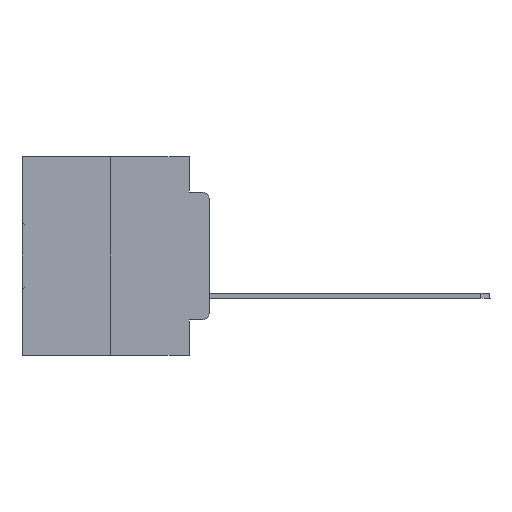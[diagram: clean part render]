
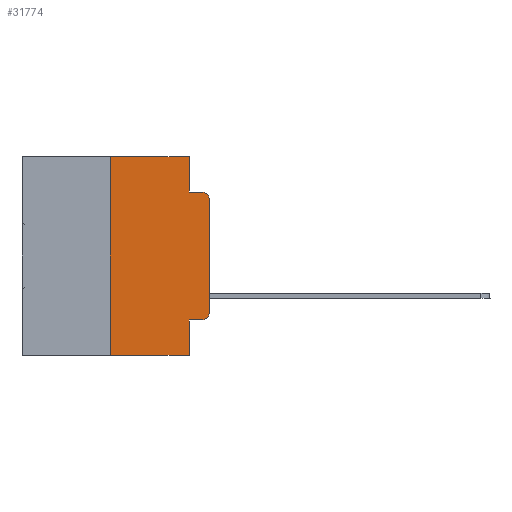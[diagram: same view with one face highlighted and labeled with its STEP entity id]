
A CAD part, left-side view. The second image highlights one B-rep face of the part: STEP entity #31774.
In plain terms, the highlighted planar face has unit normal (-1, 0, 0).
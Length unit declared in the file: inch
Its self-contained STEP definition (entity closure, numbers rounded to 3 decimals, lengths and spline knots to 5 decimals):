
#291 = CARTESIAN_POINT ( 'NONE',  ( 0., 0., -0.3915 ) ) ;
#1511 = EDGE_CURVE ( 'NONE', #17977, #1624, #19729, .T. ) ;
#1624 = VERTEX_POINT ( 'NONE', #20412 ) ;
#1772 = EDGE_LOOP ( 'NONE', ( #11025, #20666, #19394, #4101, #31444, #15307, #18161, #24381, #7701, #19922 ) ) ;
#2603 = CIRCLE ( 'NONE', #23754, 0.02 ) ;
#2684 = DIRECTION ( 'NONE',  ( 0., 0., -1. ) ) ;
#2733 = LINE ( 'NONE', #8627, #13913 ) ;
#2771 = VERTEX_POINT ( 'NONE', #5417 ) ;
#2804 = EDGE_CURVE ( 'NONE', #32951, #7761, #2733, .T. ) ;
#2939 = CARTESIAN_POINT ( 'NONE',  ( 0., 0.051, -0.4115 ) ) ;
#3077 = LINE ( 'NONE', #18173, #30361 ) ;
#3597 = DIRECTION ( 'NONE',  ( 0., -1., 0. ) ) ;
#3791 = CARTESIAN_POINT ( 'NONE',  ( 0., 0.25, 0. ) ) ;
#3848 = CARTESIAN_POINT ( 'NONE',  ( 0., 0.051, -0.5 ) ) ;
#4101 = ORIENTED_EDGE ( 'NONE', *, *, #33173, .F. ) ;
#4115 = CARTESIAN_POINT ( 'NONE',  ( 0., 0.02, -0.1085 ) ) ;
#4470 = FACE_OUTER_BOUND ( 'NONE', #1772, .T. ) ;
#4649 = EDGE_CURVE ( 'NONE', #1624, #17998, #2603, .T. ) ;
#5417 = CARTESIAN_POINT ( 'NONE',  ( 0., 0., -0.1085 ) ) ;
#6479 = LINE ( 'NONE', #16119, #21344 ) ;
#6484 = CARTESIAN_POINT ( 'NONE',  ( 0., 0.25, -0.5 ) ) ;
#6790 = CARTESIAN_POINT ( 'NONE',  ( 0., 0.051, 0. ) ) ;
#7687 = EDGE_CURVE ( 'NONE', #17998, #2771, #6479, .T. ) ;
#7701 = ORIENTED_EDGE ( 'NONE', *, *, #1511, .T. ) ;
#7761 = VERTEX_POINT ( 'NONE', #11433 ) ;
#8071 = VECTOR ( 'NONE', #3597, 39.37008 ) ;
#8291 = VERTEX_POINT ( 'NONE', #18650 ) ;
#8627 = CARTESIAN_POINT ( 'NONE',  ( 0., 0.051, -0.0885 ) ) ;
#9637 = LINE ( 'NONE', #3791, #29026 ) ;
#9749 = DIRECTION ( 'NONE',  ( 1., 0., 0. ) ) ;
#10572 = VECTOR ( 'NONE', #25533, 39.37008 ) ;
#10906 = CARTESIAN_POINT ( 'NONE',  ( 0., 0.02, -0.3915 ) ) ;
#11025 = ORIENTED_EDGE ( 'NONE', *, *, #7687, .T. ) ;
#11335 = AXIS2_PLACEMENT_3D ( 'NONE', #4115, #22582, #27676 ) ;
#11377 = CARTESIAN_POINT ( 'NONE',  ( 0., 0.473, 0. ) ) ;
#11433 = CARTESIAN_POINT ( 'NONE',  ( 0., 0.02, -0.0885 ) ) ;
#12043 = CARTESIAN_POINT ( 'NONE',  ( 0., 0.051, -0.4115 ) ) ;
#12288 = EDGE_CURVE ( 'NONE', #25626, #14626, #3077, .T. ) ;
#12292 = VECTOR ( 'NONE', #2684, 39.37008 ) ;
#13536 = DIRECTION ( 'NONE',  ( 0., 0., -1. ) ) ;
#13904 = EDGE_CURVE ( 'NONE', #25626, #8291, #9637, .T. ) ;
#13913 = VECTOR ( 'NONE', #25048, 39.37008 ) ;
#14626 = VERTEX_POINT ( 'NONE', #3848 ) ;
#15028 = CARTESIAN_POINT ( 'NONE',  ( 0., 0.473, 0. ) ) ;
#15307 = ORIENTED_EDGE ( 'NONE', *, *, #13904, .F. ) ;
#16119 = CARTESIAN_POINT ( 'NONE',  ( 0., 0., 0. ) ) ;
#17690 = DIRECTION ( 'NONE',  ( 0., 0., -1. ) ) ;
#17977 = VERTEX_POINT ( 'NONE', #2939 ) ;
#17998 = VERTEX_POINT ( 'NONE', #291 ) ;
#18161 = ORIENTED_EDGE ( 'NONE', *, *, #12288, .T. ) ;
#18173 = CARTESIAN_POINT ( 'NONE',  ( 0., 0.473, -0.5 ) ) ;
#18650 = CARTESIAN_POINT ( 'NONE',  ( 0., 0.25, 0. ) ) ;
#19394 = ORIENTED_EDGE ( 'NONE', *, *, #2804, .F. ) ;
#19729 = LINE ( 'NONE', #12043, #20132 ) ;
#19922 = ORIENTED_EDGE ( 'NONE', *, *, #4649, .T. ) ;
#20132 = VECTOR ( 'NONE', #24913, 39.37008 ) ;
#20412 = CARTESIAN_POINT ( 'NONE',  ( 0., 0.02, -0.4115 ) ) ;
#20666 = ORIENTED_EDGE ( 'NONE', *, *, #25065, .T. ) ;
#21001 = CIRCLE ( 'NONE', #11335, 0.02 ) ;
#21130 = AXIS2_PLACEMENT_3D ( 'NONE', #15028, #9749, #17690 ) ;
#21344 = VECTOR ( 'NONE', #28986, 39.37008 ) ;
#22133 = LINE ( 'NONE', #28594, #12292 ) ;
#22489 = DIRECTION ( 'NONE',  ( 0., 0., 1. ) ) ;
#22532 = CARTESIAN_POINT ( 'NONE',  ( 0., 0.051, 0. ) ) ;
#22582 = DIRECTION ( 'NONE',  ( -1., 0., 0. ) ) ;
#23754 = AXIS2_PLACEMENT_3D ( 'NONE', #10906, #32102, #13536 ) ;
#24381 = ORIENTED_EDGE ( 'NONE', *, *, #32651, .F. ) ;
#24913 = DIRECTION ( 'NONE',  ( 0., -1., 0. ) ) ;
#25048 = DIRECTION ( 'NONE',  ( 0., -1., 0. ) ) ;
#25065 = EDGE_CURVE ( 'NONE', #2771, #7761, #21001, .T. ) ;
#25533 = DIRECTION ( 'NONE',  ( 0., 0., -1. ) ) ;
#25535 = PLANE ( 'NONE',  #21130 ) ;
#25626 = VERTEX_POINT ( 'NONE', #6484 ) ;
#27141 = EDGE_CURVE ( 'NONE', #8291, #33801, #32458, .T. ) ;
#27621 = CARTESIAN_POINT ( 'NONE',  ( 0., 0.051, -0.0885 ) ) ;
#27676 = DIRECTION ( 'NONE',  ( 0., 0., -1. ) ) ;
#28594 = CARTESIAN_POINT ( 'NONE',  ( 0., 0.051, 0. ) ) ;
#28986 = DIRECTION ( 'NONE',  ( 0., 0., 1. ) ) ;
#29026 = VECTOR ( 'NONE', #22489, 39.37008 ) ;
#30361 = VECTOR ( 'NONE', #34090, 39.37008 ) ;
#31444 = ORIENTED_EDGE ( 'NONE', *, *, #27141, .F. ) ;
#31639 = LINE ( 'NONE', #22532, #10572 ) ;
#31774 = ADVANCED_FACE ( 'NONE', ( #4470 ), #25535, .F. ) ;
#32102 = DIRECTION ( 'NONE',  ( -1., 0., 0. ) ) ;
#32458 = LINE ( 'NONE', #11377, #8071 ) ;
#32651 = EDGE_CURVE ( 'NONE', #17977, #14626, #22133, .T. ) ;
#32951 = VERTEX_POINT ( 'NONE', #27621 ) ;
#33173 = EDGE_CURVE ( 'NONE', #33801, #32951, #31639, .T. ) ;
#33801 = VERTEX_POINT ( 'NONE', #6790 ) ;
#34090 = DIRECTION ( 'NONE',  ( 0., -1., 0. ) ) ;
